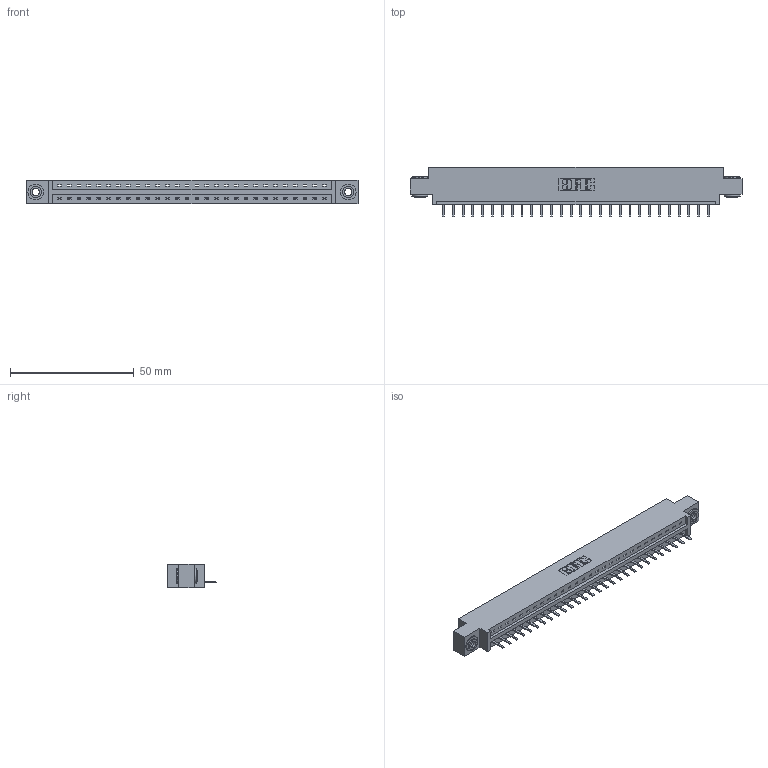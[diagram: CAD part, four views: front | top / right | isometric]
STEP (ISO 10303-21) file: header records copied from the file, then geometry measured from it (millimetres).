
FILE_DESCRIPTION (( 'STEP AP203' ), '1' );
FILE_NAME ('337-028-520-603.STEP', '2018-08-06T09:11:27', ( '' ), ( '' ), 'SwSTEP 2.0', 'SolidWorks 2016', '' );
FILE_SCHEMA (( 'CONFIG_CONTROL_DESIGN' ));
Length unit declared in the file: inch
Products named in the file (4): 337 Part_0.170 Offset - 0.156 Dia-TH; 345-292-001_345-293-120; 345-250-002_345-250-002-102; 337-028-520-603
Assembly tree (31 placements, depth 2):
  337-028-520-603
    337 Part_0.170 Offset - 0.156 Dia-TH
    345-292-001_345-293-120  x28
    345-250-002_345-250-002-102  x2
Bounding box: 133.96 x 20.02 x 9.4 mm (x, y, z)
Volume: 13569 mm3; surface area: 13983.1 mm2
Topology: 31 solids, 31 shells, 2004 faces, 5887 edges, 3846 vertices
Faces by surface type: plane 1428, cylinder 568, cone 8
Entity records: 23520 total; most frequent: CARTESIAN_POINT 4085, ORIENTED_EDGE 4030, DIRECTION 3489, EDGE_CURVE 2015, LINE 1859, VECTOR 1859, VERTEX_POINT 1338, AXIS2_PLACEMENT_3D 815
